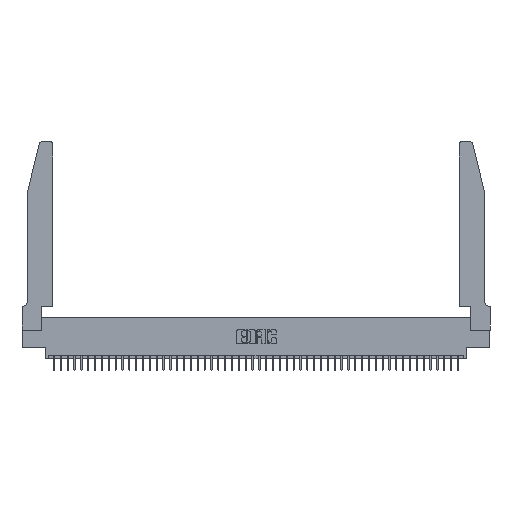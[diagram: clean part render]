
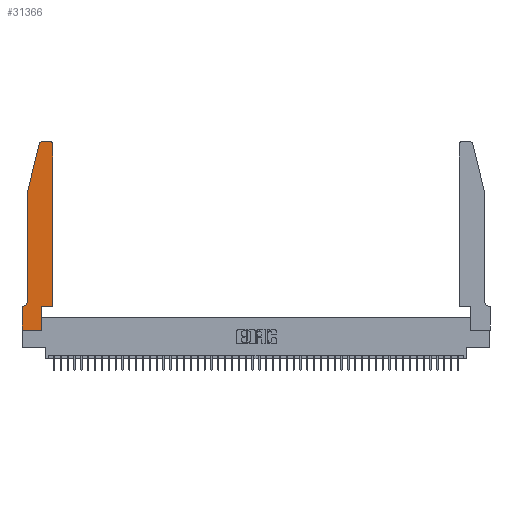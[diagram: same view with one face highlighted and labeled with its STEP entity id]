
A CAD part, top view. The second image highlights one B-rep face of the part: STEP entity #31366.
In plain terms, the highlighted planar face has unit normal (0, 0, 1).
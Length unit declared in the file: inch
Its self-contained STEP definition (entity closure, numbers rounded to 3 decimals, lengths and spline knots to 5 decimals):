
#262 = LINE ( 'NONE', #2876, #15820 ) ;
#1074 = EDGE_CURVE ( 'NONE', #18160, #7141, #44647, .T. ) ;
#1862 = VERTEX_POINT ( 'NONE', #41004 ) ;
#2876 = CARTESIAN_POINT ( 'NONE',  ( 0.0755, 0.35, 0.37 ) ) ;
#3434 = CARTESIAN_POINT ( 'NONE',  ( 0.0755, 2., 0.37 ) ) ;
#3517 = DIRECTION ( 'NONE',  ( -1., 0., 0. ) ) ;
#3642 = VERTEX_POINT ( 'NONE', #14500 ) ;
#3986 = VECTOR ( 'NONE', #5137, 39.37008 ) ;
#4393 = CARTESIAN_POINT ( 'NONE',  ( 0.2605, 2.75, 0.37 ) ) ;
#5008 = AXIS2_PLACEMENT_3D ( 'NONE', #22873, #7253, #19314 ) ;
#5137 = DIRECTION ( 'NONE',  ( 0., -1., 0. ) ) ;
#5423 = ORIENTED_EDGE ( 'NONE', *, *, #41193, .T. ) ;
#5588 = DIRECTION ( 'NONE',  ( 0., -1., 0. ) ) ;
#6360 = EDGE_LOOP ( 'NONE', ( #5423, #17095, #44288, #26583, #36098, #20788, #24975, #42761, #28468, #9182, #36685, #30741 ) ) ;
#6376 = VERTEX_POINT ( 'NONE', #14155 ) ;
#7141 = VERTEX_POINT ( 'NONE', #45964 ) ;
#7253 = DIRECTION ( 'NONE',  ( 0., 0., 1. ) ) ;
#7315 = DIRECTION ( 'NONE',  ( 0., 1., 0. ) ) ;
#7510 = CARTESIAN_POINT ( 'NONE',  ( 0.0055, 0.42, 0.37 ) ) ;
#7679 = LINE ( 'NONE', #27130, #16658 ) ;
#9026 = EDGE_CURVE ( 'NONE', #3642, #23267, #29775, .T. ) ;
#9182 = ORIENTED_EDGE ( 'NONE', *, *, #30301, .T. ) ;
#10191 = EDGE_CURVE ( 'NONE', #34322, #40399, #262, .T. ) ;
#10243 = CARTESIAN_POINT ( 'NONE',  ( 0.2865, 0.35, 0.37 ) ) ;
#11063 = AXIS2_PLACEMENT_3D ( 'NONE', #33876, #14893, #22650 ) ;
#12154 = CIRCLE ( 'NONE', #11063, 0.03 ) ;
#12562 = DIRECTION ( 'NONE',  ( -1., 0., 0. ) ) ;
#13712 = LINE ( 'NONE', #4393, #28149 ) ;
#14155 = CARTESIAN_POINT ( 'NONE',  ( 0.4205, 2.75, 0.37 ) ) ;
#14377 = CARTESIAN_POINT ( 'NONE',  ( 0.284, 2.72, 0.37 ) ) ;
#14500 = CARTESIAN_POINT ( 'NONE',  ( 0.0755, 2., 0.37 ) ) ;
#14873 = CARTESIAN_POINT ( 'NONE',  ( 0., 0., 0.37 ) ) ;
#14893 = DIRECTION ( 'NONE',  ( 0., 0., 1. ) ) ;
#15336 = DIRECTION ( 'NONE',  ( 1., 0., 0. ) ) ;
#15820 = VECTOR ( 'NONE', #22159, 39.37008 ) ;
#16308 = LINE ( 'NONE', #22778, #18134 ) ;
#16658 = VECTOR ( 'NONE', #15336, 39.37008 ) ;
#17095 = ORIENTED_EDGE ( 'NONE', *, *, #27991, .T. ) ;
#17805 = EDGE_CURVE ( 'NONE', #47897, #48203, #7679, .T. ) ;
#18134 = VECTOR ( 'NONE', #7315, 39.37008 ) ;
#18160 = VERTEX_POINT ( 'NONE', #36001 ) ;
#19314 = DIRECTION ( 'NONE',  ( 1., 0., 0. ) ) ;
#20539 = CARTESIAN_POINT ( 'NONE',  ( 0.0755, 2., 0.37 ) ) ;
#20788 = ORIENTED_EDGE ( 'NONE', *, *, #10191, .T. ) ;
#21327 = EDGE_CURVE ( 'NONE', #7141, #6376, #12154, .T. ) ;
#22131 = DIRECTION ( 'NONE',  ( 0., 0., 1. ) ) ;
#22159 = DIRECTION ( 'NONE',  ( -1., 0., 0. ) ) ;
#22548 = EDGE_CURVE ( 'NONE', #40399, #47897, #35498, .T. ) ;
#22650 = DIRECTION ( 'NONE',  ( 1., 0., 0. ) ) ;
#22778 = CARTESIAN_POINT ( 'NONE',  ( 0.2865, 0.35, 0.37 ) ) ;
#22814 = VERTEX_POINT ( 'NONE', #10243 ) ;
#22873 = CARTESIAN_POINT ( 'NONE',  ( 0., 0.35, 0.37 ) ) ;
#22886 = VECTOR ( 'NONE', #5588, 39.37008 ) ;
#23267 = VERTEX_POINT ( 'NONE', #25913 ) ;
#24428 = CARTESIAN_POINT ( 'NONE',  ( 0.2865, 0., 0.37 ) ) ;
#24975 = ORIENTED_EDGE ( 'NONE', *, *, #22548, .T. ) ;
#25652 = CIRCLE ( 'NONE', #36178, 0.07 ) ;
#25817 = CARTESIAN_POINT ( 'NONE',  ( 0.4505, 0.35, 0.37 ) ) ;
#25913 = CARTESIAN_POINT ( 'NONE',  ( 0.0755, 0.42, 0.37 ) ) ;
#26583 = ORIENTED_EDGE ( 'NONE', *, *, #9026, .T. ) ;
#26997 = CARTESIAN_POINT ( 'NONE',  ( 0.25487, 2.72718, 0.37 ) ) ;
#27130 = CARTESIAN_POINT ( 'NONE',  ( 0., 0., 0.37 ) ) ;
#27319 = CARTESIAN_POINT ( 'NONE',  ( 0.4505, 0.35, 0.37 ) ) ;
#27991 = EDGE_CURVE ( 'NONE', #1862, #30245, #29554, .T. ) ;
#28008 = LINE ( 'NONE', #3434, #41787 ) ;
#28149 = VECTOR ( 'NONE', #12562, 39.37008 ) ;
#28468 = ORIENTED_EDGE ( 'NONE', *, *, #44754, .T. ) ;
#29554 = CIRCLE ( 'NONE', #33585, 0.03 ) ;
#29703 = DIRECTION ( 'NONE',  ( 0., 1., 0. ) ) ;
#29759 = CARTESIAN_POINT ( 'NONE',  ( 0., 0., 0.37 ) ) ;
#29775 = LINE ( 'NONE', #20539, #3986 ) ;
#30245 = VERTEX_POINT ( 'NONE', #26997 ) ;
#30301 = EDGE_CURVE ( 'NONE', #22814, #18160, #37694, .T. ) ;
#30741 = ORIENTED_EDGE ( 'NONE', *, *, #21327, .T. ) ;
#30924 = DIRECTION ( 'NONE',  ( -0.239, -0.971, 0. ) ) ;
#31366 = ADVANCED_FACE ( 'NONE', ( #48941 ), #41636, .T. ) ;
#31388 = EDGE_CURVE ( 'NONE', #30245, #3642, #28008, .T. ) ;
#33254 = CARTESIAN_POINT ( 'NONE',  ( 0.0055, 0.35, 0.37 ) ) ;
#33585 = AXIS2_PLACEMENT_3D ( 'NONE', #14377, #22131, #48931 ) ;
#33876 = CARTESIAN_POINT ( 'NONE',  ( 0.4205, 2.72, 0.37 ) ) ;
#34322 = VERTEX_POINT ( 'NONE', #33254 ) ;
#34361 = DIRECTION ( 'NONE',  ( 0., 0., -1. ) ) ;
#35498 = LINE ( 'NONE', #29759, #22886 ) ;
#36001 = CARTESIAN_POINT ( 'NONE',  ( 0.4505, 0.35, 0.37 ) ) ;
#36098 = ORIENTED_EDGE ( 'NONE', *, *, #41615, .T. ) ;
#36178 = AXIS2_PLACEMENT_3D ( 'NONE', #7510, #34361, #3517 ) ;
#36685 = ORIENTED_EDGE ( 'NONE', *, *, #1074, .T. ) ;
#37694 = LINE ( 'NONE', #27319, #44276 ) ;
#38004 = CARTESIAN_POINT ( 'NONE',  ( 0., 0.35, 0.37 ) ) ;
#40399 = VERTEX_POINT ( 'NONE', #38004 ) ;
#41004 = CARTESIAN_POINT ( 'NONE',  ( 0.284, 2.75, 0.37 ) ) ;
#41193 = EDGE_CURVE ( 'NONE', #6376, #1862, #13712, .T. ) ;
#41615 = EDGE_CURVE ( 'NONE', #23267, #34322, #25652, .T. ) ;
#41636 = PLANE ( 'NONE',  #5008 ) ;
#41787 = VECTOR ( 'NONE', #30924, 39.37008 ) ;
#42761 = ORIENTED_EDGE ( 'NONE', *, *, #17805, .T. ) ;
#44276 = VECTOR ( 'NONE', #46241, 39.37008 ) ;
#44288 = ORIENTED_EDGE ( 'NONE', *, *, #31388, .T. ) ;
#44647 = LINE ( 'NONE', #25817, #49474 ) ;
#44754 = EDGE_CURVE ( 'NONE', #48203, #22814, #16308, .T. ) ;
#45964 = CARTESIAN_POINT ( 'NONE',  ( 0.4505, 2.72, 0.37 ) ) ;
#46241 = DIRECTION ( 'NONE',  ( 1., 0., 0. ) ) ;
#47897 = VERTEX_POINT ( 'NONE', #14873 ) ;
#48203 = VERTEX_POINT ( 'NONE', #24428 ) ;
#48931 = DIRECTION ( 'NONE',  ( 1., 0., 0. ) ) ;
#48941 = FACE_OUTER_BOUND ( 'NONE', #6360, .T. ) ;
#49474 = VECTOR ( 'NONE', #29703, 39.37008 ) ;
